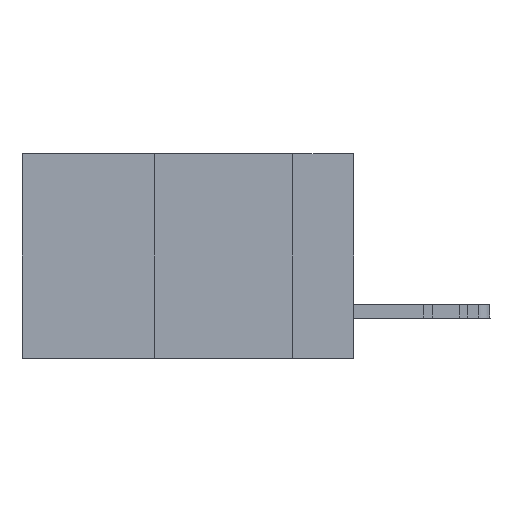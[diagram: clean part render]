
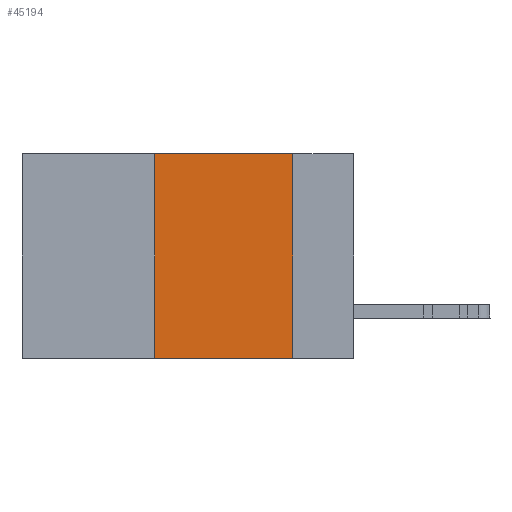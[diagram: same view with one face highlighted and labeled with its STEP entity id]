
A CAD part, left-side view. The second image highlights one B-rep face of the part: STEP entity #45194.
In plain terms, the highlighted planar face has unit normal (-1, 0, 0).
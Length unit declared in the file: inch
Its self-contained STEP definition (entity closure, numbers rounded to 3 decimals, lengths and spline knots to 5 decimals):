
#774 = VERTEX_POINT ( 'NONE', #11911 ) ;
#2003 = FACE_OUTER_BOUND ( 'NONE', #6870, .T. ) ;
#2483 = VERTEX_POINT ( 'NONE', #40143 ) ;
#4609 = DIRECTION ( 'NONE',  ( 0., -1., 0. ) ) ;
#5712 = VECTOR ( 'NONE', #4609, 39.37008 ) ;
#6848 = LINE ( 'NONE', #33080, #21337 ) ;
#6870 = EDGE_LOOP ( 'NONE', ( #24542, #36571, #44338, #9274 ) ) ;
#7841 = CARTESIAN_POINT ( 'NONE',  ( 0., 0.6, 0. ) ) ;
#8661 = VECTOR ( 'NONE', #11154, 39.37008 ) ;
#9274 = ORIENTED_EDGE ( 'NONE', *, *, #39625, .T. ) ;
#11154 = DIRECTION ( 'NONE',  ( 0., 0., 1. ) ) ;
#11911 = CARTESIAN_POINT ( 'NONE',  ( 0., 0.36, 0. ) ) ;
#13856 = CARTESIAN_POINT ( 'NONE',  ( 0., 0.11, 0. ) ) ;
#14611 = DIRECTION ( 'NONE',  ( 0., 0., -1. ) ) ;
#15346 = VERTEX_POINT ( 'NONE', #27750 ) ;
#16809 = LINE ( 'NONE', #21823, #8661 ) ;
#17107 = EDGE_CURVE ( 'NONE', #2483, #774, #16809, .T. ) ;
#18019 = PLANE ( 'NONE',  #24913 ) ;
#18185 = CARTESIAN_POINT ( 'NONE',  ( 0., 0.6, 0. ) ) ;
#21337 = VECTOR ( 'NONE', #40630, 39.37008 ) ;
#21823 = CARTESIAN_POINT ( 'NONE',  ( 0., 0.36, 0. ) ) ;
#24420 = CARTESIAN_POINT ( 'NONE',  ( 0., 0.6, -0.37 ) ) ;
#24542 = ORIENTED_EDGE ( 'NONE', *, *, #45345, .F. ) ;
#24759 = LINE ( 'NONE', #24420, #28743 ) ;
#24913 = AXIS2_PLACEMENT_3D ( 'NONE', #18185, #36464, #14611 ) ;
#27750 = CARTESIAN_POINT ( 'NONE',  ( 0., 0.11, -0.37 ) ) ;
#28743 = VECTOR ( 'NONE', #31144, 39.37008 ) ;
#29977 = LINE ( 'NONE', #7841, #5712 ) ;
#31144 = DIRECTION ( 'NONE',  ( 0., -1., 0. ) ) ;
#33015 = EDGE_CURVE ( 'NONE', #774, #34320, #29977, .T. ) ;
#33080 = CARTESIAN_POINT ( 'NONE',  ( 0., 0.11, 0. ) ) ;
#34320 = VERTEX_POINT ( 'NONE', #13856 ) ;
#36464 = DIRECTION ( 'NONE',  ( 1., 0., 0. ) ) ;
#36571 = ORIENTED_EDGE ( 'NONE', *, *, #33015, .F. ) ;
#39625 = EDGE_CURVE ( 'NONE', #2483, #15346, #24759, .T. ) ;
#40143 = CARTESIAN_POINT ( 'NONE',  ( 0., 0.36, -0.37 ) ) ;
#40630 = DIRECTION ( 'NONE',  ( 0., 0., -1. ) ) ;
#44338 = ORIENTED_EDGE ( 'NONE', *, *, #17107, .F. ) ;
#45194 = ADVANCED_FACE ( 'NONE', ( #2003 ), #18019, .F. ) ;
#45345 = EDGE_CURVE ( 'NONE', #34320, #15346, #6848, .T. ) ;
